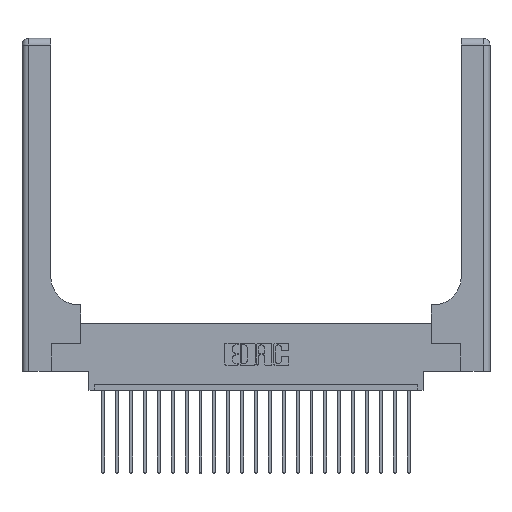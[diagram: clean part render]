
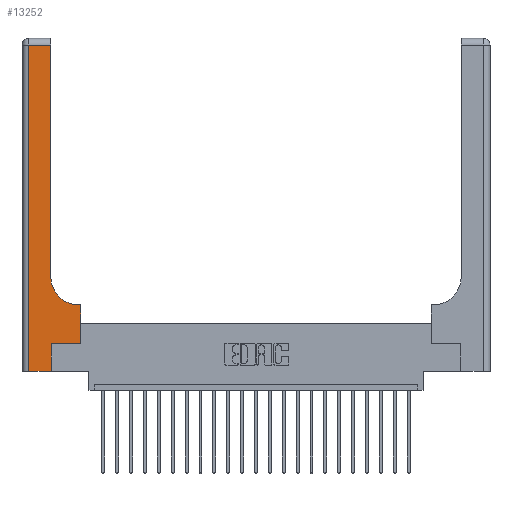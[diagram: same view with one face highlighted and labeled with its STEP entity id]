
A CAD part, top view. The second image highlights one B-rep face of the part: STEP entity #13252.
In plain terms, the highlighted planar face has unit normal (0, 0, 1).
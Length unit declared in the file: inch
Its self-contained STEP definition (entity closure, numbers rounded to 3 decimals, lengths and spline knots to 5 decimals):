
#735 = VERTEX_POINT ( 'NONE', #13933 ) ;
#1125 = FACE_OUTER_BOUND ( 'NONE', #15467, .T. ) ;
#1717 = DIRECTION ( 'NONE',  ( -1., 0., 0. ) ) ;
#1790 = EDGE_CURVE ( 'NONE', #12588, #735, #20775, .T. ) ;
#1810 = CIRCLE ( 'NONE', #14587, 0.25 ) ;
#1966 = VERTEX_POINT ( 'NONE', #4273 ) ;
#2820 = VERTEX_POINT ( 'NONE', #15505 ) ;
#3190 = CARTESIAN_POINT ( 'NONE',  ( 0.265, 0.25, 0.37 ) ) ;
#3441 = VECTOR ( 'NONE', #14777, 39.37008 ) ;
#3445 = LINE ( 'NONE', #19445, #9217 ) ;
#3664 = LINE ( 'NONE', #14190, #9963 ) ;
#3793 = VECTOR ( 'NONE', #16598, 39.37008 ) ;
#3988 = ORIENTED_EDGE ( 'NONE', *, *, #21876, .T. ) ;
#4024 = DIRECTION ( 'NONE',  ( 1., 0., 0. ) ) ;
#4273 = CARTESIAN_POINT ( 'NONE',  ( 0.265, 0., 0.37 ) ) ;
#4315 = DIRECTION ( 'NONE',  ( 1., 0., 0. ) ) ;
#4789 = CARTESIAN_POINT ( 'NONE',  ( 0., 3., 0.37 ) ) ;
#4907 = DIRECTION ( 'NONE',  ( -1., 0., 0. ) ) ;
#5146 = ORIENTED_EDGE ( 'NONE', *, *, #21644, .T. ) ;
#5244 = EDGE_CURVE ( 'NONE', #735, #1966, #18432, .T. ) ;
#5428 = VERTEX_POINT ( 'NONE', #20942 ) ;
#5574 = CARTESIAN_POINT ( 'NONE',  ( 0.51, 0.85, 0.37 ) ) ;
#5902 = DIRECTION ( 'NONE',  ( 0., 0., -1. ) ) ;
#6154 = DIRECTION ( 'NONE',  ( 0., 0., -1. ) ) ;
#6272 = LINE ( 'NONE', #13272, #3793 ) ;
#6473 = EDGE_CURVE ( 'NONE', #5428, #2820, #18555, .T. ) ;
#6850 = LINE ( 'NONE', #17288, #16713 ) ;
#7131 = CARTESIAN_POINT ( 'NONE',  ( 0.06, 3., 0.37 ) ) ;
#7139 = CARTESIAN_POINT ( 'NONE',  ( 0.51, 0.6, 0.37 ) ) ;
#8336 = PLANE ( 'NONE',  #20776 ) ;
#8929 = DIRECTION ( 'NONE',  ( 1., 0., 0. ) ) ;
#9217 = VECTOR ( 'NONE', #8929, 39.37008 ) ;
#9728 = VECTOR ( 'NONE', #17350, 39.37008 ) ;
#9736 = CARTESIAN_POINT ( 'NONE',  ( 0., 0., 0.37 ) ) ;
#9765 = EDGE_CURVE ( 'NONE', #2820, #12588, #6850, .T. ) ;
#9963 = VECTOR ( 'NONE', #20835, 39.37008 ) ;
#10203 = DIRECTION ( 'NONE',  ( 0., 1., 0. ) ) ;
#11440 = ORIENTED_EDGE ( 'NONE', *, *, #9765, .T. ) ;
#11697 = VECTOR ( 'NONE', #4024, 39.37008 ) ;
#12588 = VERTEX_POINT ( 'NONE', #19800 ) ;
#12642 = ORIENTED_EDGE ( 'NONE', *, *, #18215, .T. ) ;
#13252 = ADVANCED_FACE ( 'NONE', ( #1125 ), #8336, .F. ) ;
#13272 = CARTESIAN_POINT ( 'NONE',  ( 0.528, 0.25, 0.37 ) ) ;
#13364 = VERTEX_POINT ( 'NONE', #3190 ) ;
#13921 = VERTEX_POINT ( 'NONE', #16504 ) ;
#13933 = CARTESIAN_POINT ( 'NONE',  ( 0.06, 0., 0.37 ) ) ;
#13991 = ORIENTED_EDGE ( 'NONE', *, *, #6473, .T. ) ;
#14190 = CARTESIAN_POINT ( 'NONE',  ( 0.26, 0.6, 0.37 ) ) ;
#14587 = AXIS2_PLACEMENT_3D ( 'NONE', #5574, #5902, #4315 ) ;
#14657 = ORIENTED_EDGE ( 'NONE', *, *, #14686, .T. ) ;
#14686 = EDGE_CURVE ( 'NONE', #18725, #5428, #1810, .T. ) ;
#14777 = DIRECTION ( 'NONE',  ( 0., 1., 0. ) ) ;
#14799 = ORIENTED_EDGE ( 'NONE', *, *, #1790, .T. ) ;
#15287 = ORIENTED_EDGE ( 'NONE', *, *, #5244, .T. ) ;
#15467 = EDGE_LOOP ( 'NONE', ( #13991, #11440, #14799, #15287, #5146, #20180, #3988, #12642, #14657 ) ) ;
#15505 = CARTESIAN_POINT ( 'NONE',  ( 0.26, 2.94, 0.37 ) ) ;
#16504 = CARTESIAN_POINT ( 'NONE',  ( 0.528, 0.25, 0.37 ) ) ;
#16598 = DIRECTION ( 'NONE',  ( 0., 1., 0. ) ) ;
#16636 = VERTEX_POINT ( 'NONE', #19776 ) ;
#16713 = VECTOR ( 'NONE', #1717, 39.37008 ) ;
#17288 = CARTESIAN_POINT ( 'NONE',  ( 0., 2.94, 0.37 ) ) ;
#17350 = DIRECTION ( 'NONE',  ( 0., -1., 0. ) ) ;
#17539 = CARTESIAN_POINT ( 'NONE',  ( 0.265, 0., 0.37 ) ) ;
#18099 = CARTESIAN_POINT ( 'NONE',  ( 0.26, 3., 0.37 ) ) ;
#18215 = EDGE_CURVE ( 'NONE', #16636, #18725, #3664, .T. ) ;
#18432 = LINE ( 'NONE', #9736, #11697 ) ;
#18555 = LINE ( 'NONE', #18099, #3441 ) ;
#18725 = VERTEX_POINT ( 'NONE', #7139 ) ;
#19445 = CARTESIAN_POINT ( 'NONE',  ( 0.265, 0.25, 0.37 ) ) ;
#19644 = EDGE_CURVE ( 'NONE', #13364, #13921, #3445, .T. ) ;
#19776 = CARTESIAN_POINT ( 'NONE',  ( 0.528, 0.6, 0.37 ) ) ;
#19800 = CARTESIAN_POINT ( 'NONE',  ( 0.06, 2.94, 0.37 ) ) ;
#20180 = ORIENTED_EDGE ( 'NONE', *, *, #19644, .T. ) ;
#20738 = LINE ( 'NONE', #17539, #22421 ) ;
#20775 = LINE ( 'NONE', #7131, #9728 ) ;
#20776 = AXIS2_PLACEMENT_3D ( 'NONE', #4789, #6154, #4907 ) ;
#20835 = DIRECTION ( 'NONE',  ( -1., 0., 0. ) ) ;
#20942 = CARTESIAN_POINT ( 'NONE',  ( 0.26, 0.85, 0.37 ) ) ;
#21644 = EDGE_CURVE ( 'NONE', #1966, #13364, #20738, .T. ) ;
#21876 = EDGE_CURVE ( 'NONE', #13921, #16636, #6272, .T. ) ;
#22421 = VECTOR ( 'NONE', #10203, 39.37008 ) ;
